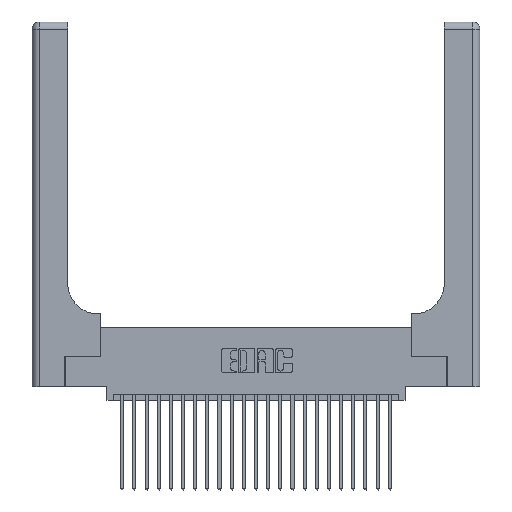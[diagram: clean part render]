
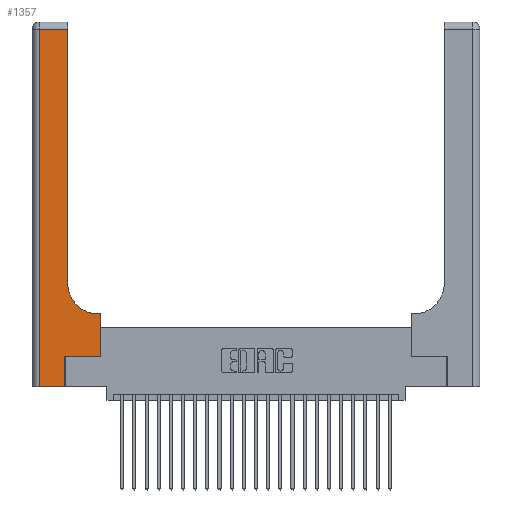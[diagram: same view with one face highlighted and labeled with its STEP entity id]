
A CAD part, top view. The second image highlights one B-rep face of the part: STEP entity #1357.
In plain terms, the highlighted planar face has unit normal (0, 0, 1).
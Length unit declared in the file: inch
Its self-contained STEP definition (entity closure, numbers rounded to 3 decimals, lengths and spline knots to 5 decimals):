
#224 = CARTESIAN_POINT ( 'NONE',  ( 0.06, 0., 0.37 ) ) ;
#293 = ORIENTED_EDGE ( 'NONE', *, *, #17973, .T. ) ;
#507 = VERTEX_POINT ( 'NONE', #224 ) ;
#1357 = ADVANCED_FACE ( 'NONE', ( #16827 ), #20584, .F. ) ;
#1639 = ORIENTED_EDGE ( 'NONE', *, *, #13647, .T. ) ;
#2076 = CARTESIAN_POINT ( 'NONE',  ( 0.2915, 0.85, 0.37 ) ) ;
#2350 = LINE ( 'NONE', #4217, #6519 ) ;
#2810 = DIRECTION ( 'NONE',  ( 0., -1., 0. ) ) ;
#2975 = ORIENTED_EDGE ( 'NONE', *, *, #6875, .T. ) ;
#3467 = CARTESIAN_POINT ( 'NONE',  ( 0.5585, 0.25, 0.37 ) ) ;
#4217 = CARTESIAN_POINT ( 'NONE',  ( 0.2915, 3., 0.37 ) ) ;
#4263 = ORIENTED_EDGE ( 'NONE', *, *, #10201, .T. ) ;
#4458 = DIRECTION ( 'NONE',  ( -1., 0., 0. ) ) ;
#5007 = LINE ( 'NONE', #19718, #20818 ) ;
#5149 = CARTESIAN_POINT ( 'NONE',  ( 0.2915, 0.6, 0.37 ) ) ;
#5553 = ORIENTED_EDGE ( 'NONE', *, *, #21938, .T. ) ;
#5733 = EDGE_CURVE ( 'NONE', #8604, #13424, #11476, .T. ) ;
#5978 = VECTOR ( 'NONE', #9753, 39.37008 ) ;
#6253 = DIRECTION ( 'NONE',  ( 0., 1., 0. ) ) ;
#6519 = VECTOR ( 'NONE', #6253, 39.37008 ) ;
#6875 = EDGE_CURVE ( 'NONE', #15990, #19032, #12340, .T. ) ;
#6899 = CARTESIAN_POINT ( 'NONE',  ( 0.06, 3., 0.37 ) ) ;
#6958 = VERTEX_POINT ( 'NONE', #21414 ) ;
#7008 = LINE ( 'NONE', #20264, #12379 ) ;
#7108 = VERTEX_POINT ( 'NONE', #25758 ) ;
#7448 = CARTESIAN_POINT ( 'NONE',  ( 0.269, 0., 0.37 ) ) ;
#8370 = AXIS2_PLACEMENT_3D ( 'NONE', #20312, #20187, #20155 ) ;
#8435 = DIRECTION ( 'NONE',  ( 0., 1., 0. ) ) ;
#8604 = VERTEX_POINT ( 'NONE', #11296 ) ;
#8775 = EDGE_LOOP ( 'NONE', ( #293, #17061, #1639, #22914, #2975, #4263, #9679, #5553, #16164 ) ) ;
#9187 = AXIS2_PLACEMENT_3D ( 'NONE', #23387, #11625, #25380 ) ;
#9679 = ORIENTED_EDGE ( 'NONE', *, *, #21203, .T. ) ;
#9725 = VECTOR ( 'NONE', #4458, 39.37008 ) ;
#9753 = DIRECTION ( 'NONE',  ( 1., 0., 0. ) ) ;
#10201 = EDGE_CURVE ( 'NONE', #19032, #11233, #5007, .T. ) ;
#11233 = VERTEX_POINT ( 'NONE', #3467 ) ;
#11296 = CARTESIAN_POINT ( 'NONE',  ( 0.5415, 0.6, 0.37 ) ) ;
#11351 = LINE ( 'NONE', #13641, #5978 ) ;
#11399 = DIRECTION ( 'NONE',  ( 0., 1., 0. ) ) ;
#11412 = LINE ( 'NONE', #5149, #16018 ) ;
#11476 = CIRCLE ( 'NONE', #9187, 0.25 ) ;
#11625 = DIRECTION ( 'NONE',  ( 0., 0., -1. ) ) ;
#12340 = LINE ( 'NONE', #25146, #22140 ) ;
#12372 = VERTEX_POINT ( 'NONE', #16629 ) ;
#12379 = VECTOR ( 'NONE', #8435, 39.37008 ) ;
#13424 = VERTEX_POINT ( 'NONE', #2076 ) ;
#13641 = CARTESIAN_POINT ( 'NONE',  ( 0., 0., 0.37 ) ) ;
#13647 = EDGE_CURVE ( 'NONE', #6958, #507, #15489, .T. ) ;
#15489 = LINE ( 'NONE', #6899, #20678 ) ;
#15990 = VERTEX_POINT ( 'NONE', #7448 ) ;
#16018 = VECTOR ( 'NONE', #24997, 39.37008 ) ;
#16164 = ORIENTED_EDGE ( 'NONE', *, *, #5733, .T. ) ;
#16618 = EDGE_CURVE ( 'NONE', #507, #15990, #11351, .T. ) ;
#16629 = CARTESIAN_POINT ( 'NONE',  ( 0.5585, 0.6, 0.37 ) ) ;
#16827 = FACE_OUTER_BOUND ( 'NONE', #8775, .T. ) ;
#17061 = ORIENTED_EDGE ( 'NONE', *, *, #25035, .T. ) ;
#17973 = EDGE_CURVE ( 'NONE', #13424, #7108, #2350, .T. ) ;
#19032 = VERTEX_POINT ( 'NONE', #21358 ) ;
#19718 = CARTESIAN_POINT ( 'NONE',  ( 0.269, 0.25, 0.37 ) ) ;
#20155 = DIRECTION ( 'NONE',  ( -1., 0., 0. ) ) ;
#20187 = DIRECTION ( 'NONE',  ( 0., 0., -1. ) ) ;
#20264 = CARTESIAN_POINT ( 'NONE',  ( 0.5585, 0.25, 0.37 ) ) ;
#20312 = CARTESIAN_POINT ( 'NONE',  ( 0., 3., 0.37 ) ) ;
#20584 = PLANE ( 'NONE',  #8370 ) ;
#20678 = VECTOR ( 'NONE', #2810, 39.37008 ) ;
#20777 = LINE ( 'NONE', #22342, #9725 ) ;
#20818 = VECTOR ( 'NONE', #21684, 39.37008 ) ;
#21203 = EDGE_CURVE ( 'NONE', #11233, #12372, #7008, .T. ) ;
#21358 = CARTESIAN_POINT ( 'NONE',  ( 0.269, 0.25, 0.37 ) ) ;
#21414 = CARTESIAN_POINT ( 'NONE',  ( 0.06, 2.94, 0.37 ) ) ;
#21684 = DIRECTION ( 'NONE',  ( 1., 0., 0. ) ) ;
#21938 = EDGE_CURVE ( 'NONE', #12372, #8604, #11412, .T. ) ;
#22140 = VECTOR ( 'NONE', #11399, 39.37008 ) ;
#22342 = CARTESIAN_POINT ( 'NONE',  ( 0., 2.94, 0.37 ) ) ;
#22914 = ORIENTED_EDGE ( 'NONE', *, *, #16618, .T. ) ;
#23387 = CARTESIAN_POINT ( 'NONE',  ( 0.5415, 0.85, 0.37 ) ) ;
#24997 = DIRECTION ( 'NONE',  ( -1., 0., 0. ) ) ;
#25035 = EDGE_CURVE ( 'NONE', #7108, #6958, #20777, .T. ) ;
#25146 = CARTESIAN_POINT ( 'NONE',  ( 0.269, 0., 0.37 ) ) ;
#25380 = DIRECTION ( 'NONE',  ( 1., 0., 0. ) ) ;
#25758 = CARTESIAN_POINT ( 'NONE',  ( 0.2915, 2.94, 0.37 ) ) ;
